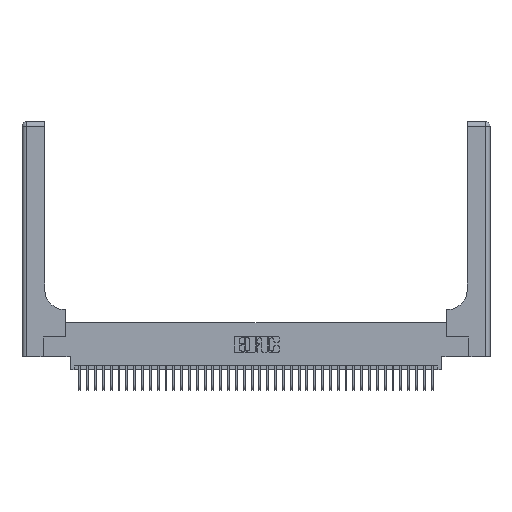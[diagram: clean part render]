
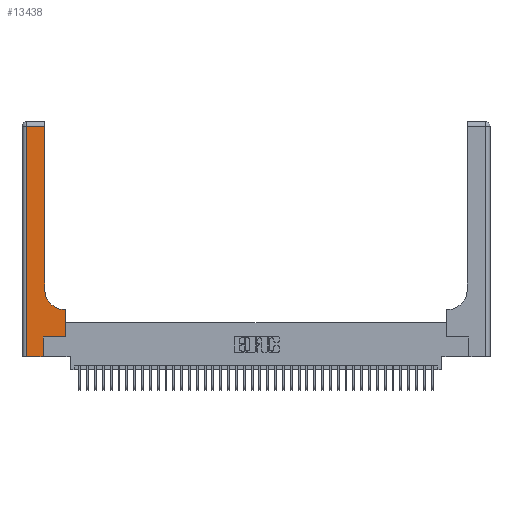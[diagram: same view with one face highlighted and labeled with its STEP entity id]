
A CAD part, top view. The second image highlights one B-rep face of the part: STEP entity #13438.
In plain terms, the highlighted planar face has unit normal (0, 0, 1).
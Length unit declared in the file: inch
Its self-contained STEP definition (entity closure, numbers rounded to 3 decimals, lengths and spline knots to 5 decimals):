
#217 = CARTESIAN_POINT ( 'NONE',  ( 0.5585, 0.25, 0.37 ) ) ;
#1162 = CARTESIAN_POINT ( 'NONE',  ( 0.269, 0.25, 0.37 ) ) ;
#1401 = DIRECTION ( 'NONE',  ( -1., 0., 0. ) ) ;
#1402 = CARTESIAN_POINT ( 'NONE',  ( 0.269, 0., 0.37 ) ) ;
#1843 = VECTOR ( 'NONE', #17974, 39.37008 ) ;
#2729 = LINE ( 'NONE', #217, #34272 ) ;
#2770 = VECTOR ( 'NONE', #3451, 39.37008 ) ;
#3451 = DIRECTION ( 'NONE',  ( -1., 0., 0. ) ) ;
#3614 = VERTEX_POINT ( 'NONE', #30954 ) ;
#3802 = VERTEX_POINT ( 'NONE', #13514 ) ;
#4584 = VECTOR ( 'NONE', #28303, 39.37008 ) ;
#4607 = CARTESIAN_POINT ( 'NONE',  ( 0.2915, 0.6, 0.37 ) ) ;
#6075 = EDGE_CURVE ( 'NONE', #6514, #3614, #24858, .T. ) ;
#6286 = EDGE_CURVE ( 'NONE', #12156, #21071, #33414, .T. ) ;
#6514 = VERTEX_POINT ( 'NONE', #13022 ) ;
#6817 = EDGE_CURVE ( 'NONE', #10197, #12156, #39448, .T. ) ;
#7073 = VECTOR ( 'NONE', #11642, 39.37008 ) ;
#7898 = CARTESIAN_POINT ( 'NONE',  ( 0.5585, 0.25, 0.37 ) ) ;
#7987 = EDGE_CURVE ( 'NONE', #8787, #6514, #37544, .T. ) ;
#8701 = CARTESIAN_POINT ( 'NONE',  ( 0.269, 0., 0.37 ) ) ;
#8787 = VERTEX_POINT ( 'NONE', #39019 ) ;
#8988 = EDGE_CURVE ( 'NONE', #39384, #3802, #35243, .T. ) ;
#9146 = VECTOR ( 'NONE', #28285, 39.37008 ) ;
#10197 = VERTEX_POINT ( 'NONE', #25068 ) ;
#10267 = EDGE_CURVE ( 'NONE', #3614, #39384, #12775, .T. ) ;
#10857 = DIRECTION ( 'NONE',  ( 0., -1., 0. ) ) ;
#10865 = CARTESIAN_POINT ( 'NONE',  ( 0.5415, 0.85, 0.37 ) ) ;
#11642 = DIRECTION ( 'NONE',  ( 1., 0., 0. ) ) ;
#12156 = VERTEX_POINT ( 'NONE', #1402 ) ;
#12775 = LINE ( 'NONE', #22152, #4584 ) ;
#12948 = VERTEX_POINT ( 'NONE', #7898 ) ;
#13022 = CARTESIAN_POINT ( 'NONE',  ( 0.5415, 0.6, 0.37 ) ) ;
#13325 = VECTOR ( 'NONE', #1401, 39.37008 ) ;
#13438 = ADVANCED_FACE ( 'NONE', ( #28325 ), #32571, .F. ) ;
#13514 = CARTESIAN_POINT ( 'NONE',  ( 0.06, 2.94, 0.37 ) ) ;
#13993 = DIRECTION ( 'NONE',  ( 1., 0., 0. ) ) ;
#14326 = CARTESIAN_POINT ( 'NONE',  ( 0., 3., 0.37 ) ) ;
#14396 = ORIENTED_EDGE ( 'NONE', *, *, #6286, .T. ) ;
#15211 = AXIS2_PLACEMENT_3D ( 'NONE', #14326, #35591, #17384 ) ;
#16834 = AXIS2_PLACEMENT_3D ( 'NONE', #10865, #32251, #13993 ) ;
#17384 = DIRECTION ( 'NONE',  ( -1., 0., 0. ) ) ;
#17642 = ORIENTED_EDGE ( 'NONE', *, *, #23938, .T. ) ;
#17751 = EDGE_CURVE ( 'NONE', #3802, #10197, #35878, .T. ) ;
#17974 = DIRECTION ( 'NONE',  ( 0., 1., 0. ) ) ;
#18140 = ORIENTED_EDGE ( 'NONE', *, *, #10267, .T. ) ;
#21071 = VERTEX_POINT ( 'NONE', #1162 ) ;
#21991 = ORIENTED_EDGE ( 'NONE', *, *, #7987, .T. ) ;
#22152 = CARTESIAN_POINT ( 'NONE',  ( 0.2915, 3., 0.37 ) ) ;
#22526 = ORIENTED_EDGE ( 'NONE', *, *, #30336, .T. ) ;
#23790 = CARTESIAN_POINT ( 'NONE',  ( 0., 0., 0.37 ) ) ;
#23938 = EDGE_CURVE ( 'NONE', #21071, #12948, #26390, .T. ) ;
#24858 = CIRCLE ( 'NONE', #16834, 0.25 ) ;
#25068 = CARTESIAN_POINT ( 'NONE',  ( 0.06, 0., 0.37 ) ) ;
#26390 = LINE ( 'NONE', #34238, #9146 ) ;
#27840 = VECTOR ( 'NONE', #10857, 39.37008 ) ;
#28285 = DIRECTION ( 'NONE',  ( 1., 0., 0. ) ) ;
#28303 = DIRECTION ( 'NONE',  ( 0., 1., 0. ) ) ;
#28325 = FACE_OUTER_BOUND ( 'NONE', #38557, .T. ) ;
#28682 = ORIENTED_EDGE ( 'NONE', *, *, #6075, .T. ) ;
#30336 = EDGE_CURVE ( 'NONE', #12948, #8787, #2729, .T. ) ;
#30851 = DIRECTION ( 'NONE',  ( 0., 1., 0. ) ) ;
#30954 = CARTESIAN_POINT ( 'NONE',  ( 0.2915, 0.85, 0.37 ) ) ;
#30981 = CARTESIAN_POINT ( 'NONE',  ( 0., 2.94, 0.37 ) ) ;
#32243 = CARTESIAN_POINT ( 'NONE',  ( 0.06, 3., 0.37 ) ) ;
#32251 = DIRECTION ( 'NONE',  ( 0., 0., -1. ) ) ;
#32571 = PLANE ( 'NONE',  #15211 ) ;
#32974 = ORIENTED_EDGE ( 'NONE', *, *, #17751, .T. ) ;
#33414 = LINE ( 'NONE', #8701, #1843 ) ;
#33803 = CARTESIAN_POINT ( 'NONE',  ( 0.2915, 2.94, 0.37 ) ) ;
#34238 = CARTESIAN_POINT ( 'NONE',  ( 0.269, 0.25, 0.37 ) ) ;
#34272 = VECTOR ( 'NONE', #30851, 39.37008 ) ;
#35243 = LINE ( 'NONE', #30981, #2770 ) ;
#35591 = DIRECTION ( 'NONE',  ( 0., 0., -1. ) ) ;
#35878 = LINE ( 'NONE', #32243, #27840 ) ;
#37544 = LINE ( 'NONE', #4607, #13325 ) ;
#38557 = EDGE_LOOP ( 'NONE', ( #18140, #39089, #32974, #38817, #14396, #17642, #22526, #21991, #28682 ) ) ;
#38817 = ORIENTED_EDGE ( 'NONE', *, *, #6817, .T. ) ;
#39019 = CARTESIAN_POINT ( 'NONE',  ( 0.5585, 0.6, 0.37 ) ) ;
#39089 = ORIENTED_EDGE ( 'NONE', *, *, #8988, .T. ) ;
#39384 = VERTEX_POINT ( 'NONE', #33803 ) ;
#39448 = LINE ( 'NONE', #23790, #7073 ) ;
